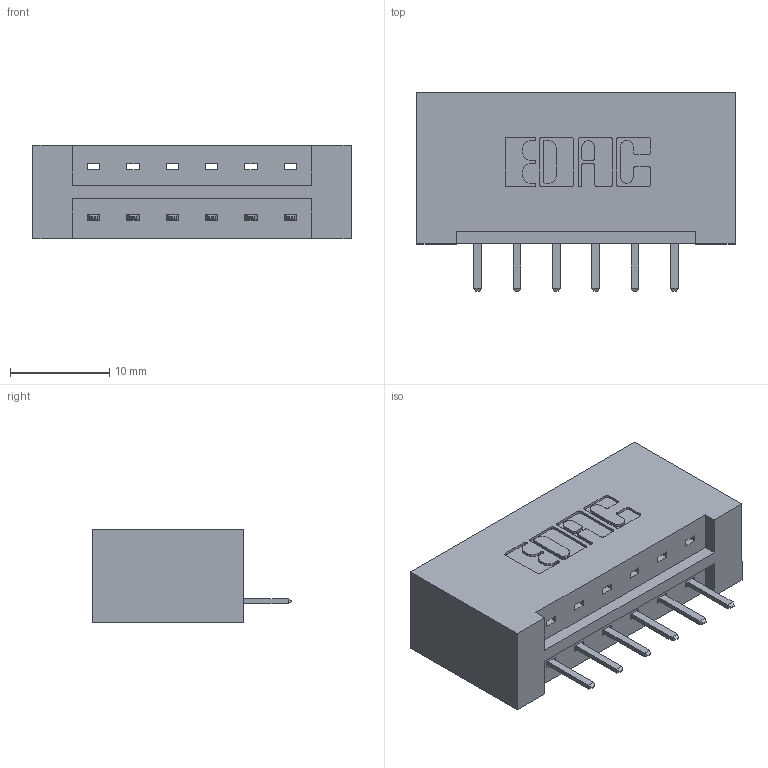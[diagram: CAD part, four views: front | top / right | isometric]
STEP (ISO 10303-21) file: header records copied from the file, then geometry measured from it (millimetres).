
FILE_DESCRIPTION (( 'STEP AP203' ), '1' );
FILE_NAME ('833-006-520-101.STEP', '2020-05-30T13:19:08', ( '' ), ( '' ), 'SwSTEP 2.0', 'SolidWorks 2020', '' );
FILE_SCHEMA (( 'CONFIG_CONTROL_DESIGN' ));
Length unit declared in the file: inch
Products named in the file (3): 833 Part_Lugless; 345-292-001_345-293-120; 833-006-520-101
Assembly tree (7 placements, depth 2):
  833-006-520-101
    833 Part_Lugless
    345-292-001_345-293-120  x6
Bounding box: 32.03 x 20.02 x 9.4 mm (x, y, z)
Volume: 3509 mm3; surface area: 3456.9 mm2
Topology: 7 solids, 7 shells, 478 faces, 1391 edges, 910 vertices
Faces by surface type: plane 330, cylinder 148
Entity records: 8161 total; most frequent: CARTESIAN_POINT 1432, ORIENTED_EDGE 1362, DIRECTION 1261, EDGE_CURVE 681, LINE 557, VECTOR 557, VERTEX_POINT 450, AXIS2_PLACEMENT_3D 352
